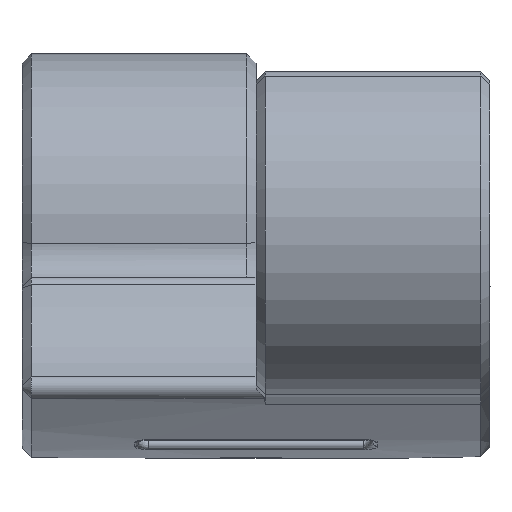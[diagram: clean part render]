
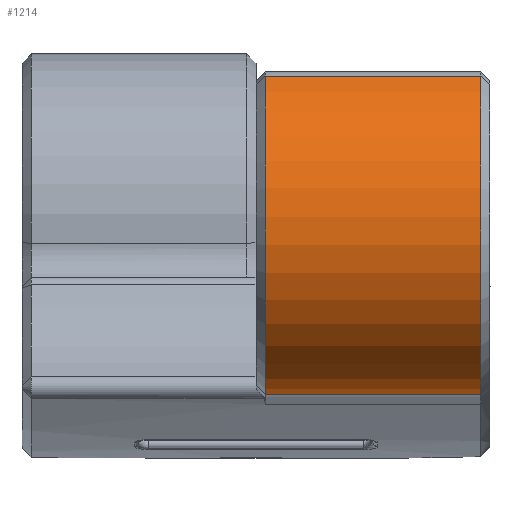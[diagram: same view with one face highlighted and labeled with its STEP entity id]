
A CAD part, front view. The second image highlights one B-rep face of the part: STEP entity #1214.
In plain terms, the highlighted cylindrical face has radius 14.583 mm (diameter 29.165 mm), a partial arc.
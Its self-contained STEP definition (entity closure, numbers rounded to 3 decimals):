
#73 = CARTESIAN_POINT ( 'NONE',  ( -459.696, -69.39, -13.751 ) ) ;
#81 = DIRECTION ( 'NONE',  ( 1., 0., 0. ) ) ;
#429 = EDGE_CURVE ( 'NONE', #869, #2937, #762, .T. ) ;
#569 = AXIS2_PLACEMENT_3D ( 'NONE', #658, #3499, #1609 ) ;
#580 = VECTOR ( 'NONE', #2889, 1000. ) ;
#632 = AXIS2_PLACEMENT_3D ( 'NONE', #2931, #81, #3220 ) ;
#658 = CARTESIAN_POINT ( 'NONE',  ( -459.696, -70.336, 0.8 ) ) ;
#762 = CIRCLE ( 'NONE', #3003, 14.583 ) ;
#843 = LINE ( 'NONE', #889, #580 ) ;
#869 = VERTEX_POINT ( 'NONE', #1934 ) ;
#889 = CARTESIAN_POINT ( 'NONE',  ( -459.696, -77.575, 13.459 ) ) ;
#1045 = DIRECTION ( 'NONE',  ( 0., 0., -1. ) ) ;
#1214 = ADVANCED_FACE ( 'NONE', ( #3462 ), #2925, .T. ) ;
#1414 = EDGE_CURVE ( 'NONE', #1600, #869, #2162, .T. ) ;
#1600 = VERTEX_POINT ( 'NONE', #2852 ) ;
#1609 = DIRECTION ( 'NONE',  ( 0., -0.958, -0.288 ) ) ;
#1611 = CIRCLE ( 'NONE', #632, 14.583 ) ;
#1795 = CARTESIAN_POINT ( 'NONE',  ( -443.881, -77.575, 13.459 ) ) ;
#1810 = VERTEX_POINT ( 'NONE', #1943 ) ;
#1821 = EDGE_LOOP ( 'NONE', ( #2866, #3378, #3506, #2629 ) ) ;
#1873 = DIRECTION ( 'NONE',  ( -1., 0., 0. ) ) ;
#1934 = CARTESIAN_POINT ( 'NONE',  ( -443.881, -69.39, -13.751 ) ) ;
#1943 = CARTESIAN_POINT ( 'NONE',  ( -425.481, -77.575, 13.459 ) ) ;
#2162 = LINE ( 'NONE', #73, #3502 ) ;
#2200 = CARTESIAN_POINT ( 'NONE',  ( -443.881, -70.336, 0.8 ) ) ;
#2629 = ORIENTED_EDGE ( 'NONE', *, *, #2829, .F. ) ;
#2829 = EDGE_CURVE ( 'NONE', #2937, #1810, #843, .T. ) ;
#2852 = CARTESIAN_POINT ( 'NONE',  ( -425.481, -69.39, -13.751 ) ) ;
#2866 = ORIENTED_EDGE ( 'NONE', *, *, #429, .F. ) ;
#2889 = DIRECTION ( 'NONE',  ( 1., 0., 0. ) ) ;
#2925 = CYLINDRICAL_SURFACE ( 'NONE', #569, 14.583 ) ;
#2931 = CARTESIAN_POINT ( 'NONE',  ( -425.481, -70.336, 0.8 ) ) ;
#2937 = VERTEX_POINT ( 'NONE', #1795 ) ;
#3003 = AXIS2_PLACEMENT_3D ( 'NONE', #2200, #3580, #1045 ) ;
#3220 = DIRECTION ( 'NONE',  ( 0., 0., -1. ) ) ;
#3349 = EDGE_CURVE ( 'NONE', #1810, #1600, #1611, .T. ) ;
#3378 = ORIENTED_EDGE ( 'NONE', *, *, #1414, .F. ) ;
#3462 = FACE_OUTER_BOUND ( 'NONE', #1821, .T. ) ;
#3499 = DIRECTION ( 'NONE',  ( 1., 0., 0. ) ) ;
#3502 = VECTOR ( 'NONE', #1873, 1000. ) ;
#3506 = ORIENTED_EDGE ( 'NONE', *, *, #3349, .F. ) ;
#3580 = DIRECTION ( 'NONE',  ( -1., 0., 0. ) ) ;
